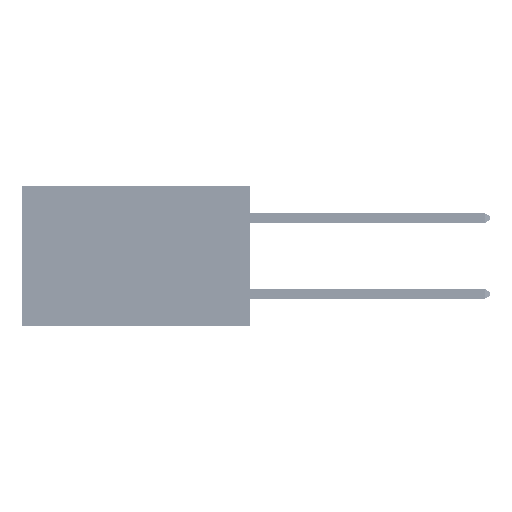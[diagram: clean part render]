
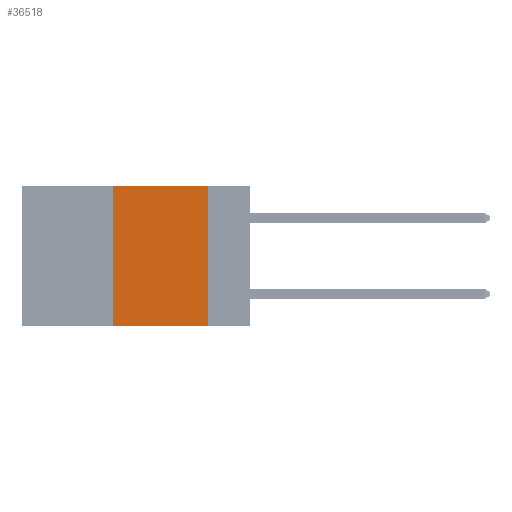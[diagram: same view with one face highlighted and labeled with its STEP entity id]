
A CAD part, left-side view. The second image highlights one B-rep face of the part: STEP entity #36518.
In plain terms, the highlighted planar face has unit normal (-1, 0, 0).
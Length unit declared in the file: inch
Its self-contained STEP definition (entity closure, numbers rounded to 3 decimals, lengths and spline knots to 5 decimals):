
#427 = VERTEX_POINT ( 'NONE', #44478 ) ;
#1257 = EDGE_CURVE ( 'NONE', #427, #9642, #33347, .T. ) ;
#1353 = FACE_OUTER_BOUND ( 'NONE', #30316, .T. ) ;
#1759 = CARTESIAN_POINT ( 'NONE',  ( 0., 0.11, 0. ) ) ;
#1780 = CARTESIAN_POINT ( 'NONE',  ( 0., 0.36, 0. ) ) ;
#5360 = VECTOR ( 'NONE', #14055, 39.37008 ) ;
#8981 = CARTESIAN_POINT ( 'NONE',  ( 0., 0.6, -0.37 ) ) ;
#9642 = VERTEX_POINT ( 'NONE', #12366 ) ;
#10349 = VECTOR ( 'NONE', #46345, 39.37008 ) ;
#12366 = CARTESIAN_POINT ( 'NONE',  ( 0., 0.36, 0. ) ) ;
#12752 = AXIS2_PLACEMENT_3D ( 'NONE', #13038, #46063, #25443 ) ;
#13038 = CARTESIAN_POINT ( 'NONE',  ( 0., 0.6, 0. ) ) ;
#14055 = DIRECTION ( 'NONE',  ( 0., 0., 1. ) ) ;
#14229 = LINE ( 'NONE', #8981, #30715 ) ;
#14937 = CARTESIAN_POINT ( 'NONE',  ( 0., 0.11, 0. ) ) ;
#15848 = LINE ( 'NONE', #1759, #18974 ) ;
#17693 = ORIENTED_EDGE ( 'NONE', *, *, #24222, .F. ) ;
#17932 = CARTESIAN_POINT ( 'NONE',  ( 0., 0.6, 0. ) ) ;
#18974 = VECTOR ( 'NONE', #34785, 39.37008 ) ;
#19464 = ORIENTED_EDGE ( 'NONE', *, *, #49131, .T. ) ;
#21367 = PLANE ( 'NONE',  #12752 ) ;
#21633 = CARTESIAN_POINT ( 'NONE',  ( 0., 0.11, -0.37 ) ) ;
#24222 = EDGE_CURVE ( 'NONE', #9642, #34169, #39608, .T. ) ;
#25443 = DIRECTION ( 'NONE',  ( 0., 0., -1. ) ) ;
#25486 = DIRECTION ( 'NONE',  ( 0., -1., 0. ) ) ;
#30034 = VERTEX_POINT ( 'NONE', #21633 ) ;
#30316 = EDGE_LOOP ( 'NONE', ( #31917, #17693, #49754, #19464 ) ) ;
#30715 = VECTOR ( 'NONE', #25486, 39.37008 ) ;
#31917 = ORIENTED_EDGE ( 'NONE', *, *, #45481, .F. ) ;
#33347 = LINE ( 'NONE', #1780, #5360 ) ;
#34169 = VERTEX_POINT ( 'NONE', #14937 ) ;
#34785 = DIRECTION ( 'NONE',  ( 0., 0., -1. ) ) ;
#36518 = ADVANCED_FACE ( 'NONE', ( #1353 ), #21367, .F. ) ;
#39608 = LINE ( 'NONE', #17932, #10349 ) ;
#44478 = CARTESIAN_POINT ( 'NONE',  ( 0., 0.36, -0.37 ) ) ;
#45481 = EDGE_CURVE ( 'NONE', #34169, #30034, #15848, .T. ) ;
#46063 = DIRECTION ( 'NONE',  ( 1., 0., 0. ) ) ;
#46345 = DIRECTION ( 'NONE',  ( 0., -1., 0. ) ) ;
#49131 = EDGE_CURVE ( 'NONE', #427, #30034, #14229, .T. ) ;
#49754 = ORIENTED_EDGE ( 'NONE', *, *, #1257, .F. ) ;
